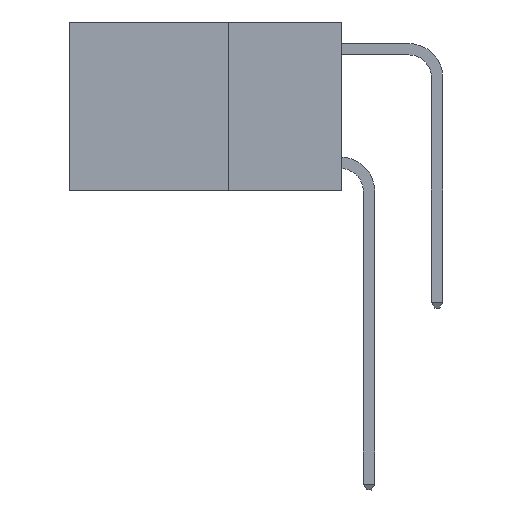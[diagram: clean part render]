
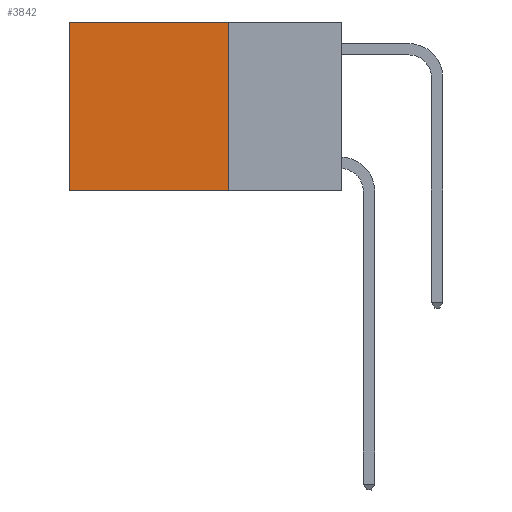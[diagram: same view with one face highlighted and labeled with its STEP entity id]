
A CAD part, left-side view. The second image highlights one B-rep face of the part: STEP entity #3842.
In plain terms, the highlighted planar face has unit normal (-1, 0, 0).
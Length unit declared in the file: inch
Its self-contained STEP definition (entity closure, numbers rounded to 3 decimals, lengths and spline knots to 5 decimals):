
#147 = DIRECTION ( 'NONE',  ( 0., 0., -1. ) ) ;
#222 = FACE_OUTER_BOUND ( 'NONE', #11064, .T. ) ;
#544 = LINE ( 'NONE', #8519, #2280 ) ;
#912 = DIRECTION ( 'NONE',  ( 0., 0., -1. ) ) ;
#1098 = DIRECTION ( 'NONE',  ( 1., 0., 0. ) ) ;
#1777 = CARTESIAN_POINT ( 'NONE',  ( 0.2625, 0.25, 0. ) ) ;
#2071 = VERTEX_POINT ( 'NONE', #6947 ) ;
#2124 = VECTOR ( 'NONE', #912, 39.37008 ) ;
#2280 = VECTOR ( 'NONE', #8874, 39.37008 ) ;
#2288 = CARTESIAN_POINT ( 'NONE',  ( 0.2625, 0.25, 0. ) ) ;
#2628 = CARTESIAN_POINT ( 'NONE',  ( 0.2625, 0.25, -0.37 ) ) ;
#2980 = AXIS2_PLACEMENT_3D ( 'NONE', #2288, #1098, #147 ) ;
#3039 = LINE ( 'NONE', #1777, #8284 ) ;
#3842 = ADVANCED_FACE ( 'NONE', ( #222 ), #7013, .F. ) ;
#3981 = VERTEX_POINT ( 'NONE', #9866 ) ;
#4516 = ORIENTED_EDGE ( 'NONE', *, *, #14330, .F. ) ;
#4647 = ORIENTED_EDGE ( 'NONE', *, *, #6139, .T. ) ;
#5881 = LINE ( 'NONE', #2628, #7530 ) ;
#6139 = EDGE_CURVE ( 'NONE', #7485, #6390, #544, .T. ) ;
#6390 = VERTEX_POINT ( 'NONE', #9247 ) ;
#6781 = EDGE_CURVE ( 'NONE', #2071, #3981, #5881, .T. ) ;
#6947 = CARTESIAN_POINT ( 'NONE',  ( 0.2625, 0.25, -0.37 ) ) ;
#7013 = PLANE ( 'NONE',  #2980 ) ;
#7485 = VERTEX_POINT ( 'NONE', #8373 ) ;
#7530 = VECTOR ( 'NONE', #13924, 39.37008 ) ;
#8284 = VECTOR ( 'NONE', #12979, 39.37008 ) ;
#8373 = CARTESIAN_POINT ( 'NONE',  ( 0.2625, 0.25, 0. ) ) ;
#8519 = CARTESIAN_POINT ( 'NONE',  ( 0.2625, 0.25, 0. ) ) ;
#8874 = DIRECTION ( 'NONE',  ( 0., 1., 0. ) ) ;
#8908 = LINE ( 'NONE', #11080, #2124 ) ;
#9247 = CARTESIAN_POINT ( 'NONE',  ( 0.2625, 0.6, 0. ) ) ;
#9866 = CARTESIAN_POINT ( 'NONE',  ( 0.2625, 0.6, -0.37 ) ) ;
#11064 = EDGE_LOOP ( 'NONE', ( #13130, #11604, #4516, #4647 ) ) ;
#11080 = CARTESIAN_POINT ( 'NONE',  ( 0.2625, 0.6, 0. ) ) ;
#11604 = ORIENTED_EDGE ( 'NONE', *, *, #6781, .F. ) ;
#12979 = DIRECTION ( 'NONE',  ( 0., 0., -1. ) ) ;
#13130 = ORIENTED_EDGE ( 'NONE', *, *, #14103, .T. ) ;
#13924 = DIRECTION ( 'NONE',  ( 0., 1., 0. ) ) ;
#14103 = EDGE_CURVE ( 'NONE', #6390, #3981, #8908, .T. ) ;
#14330 = EDGE_CURVE ( 'NONE', #7485, #2071, #3039, .T. ) ;
